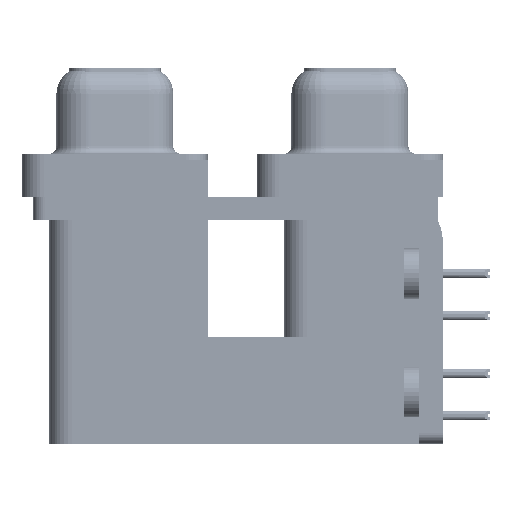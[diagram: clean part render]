
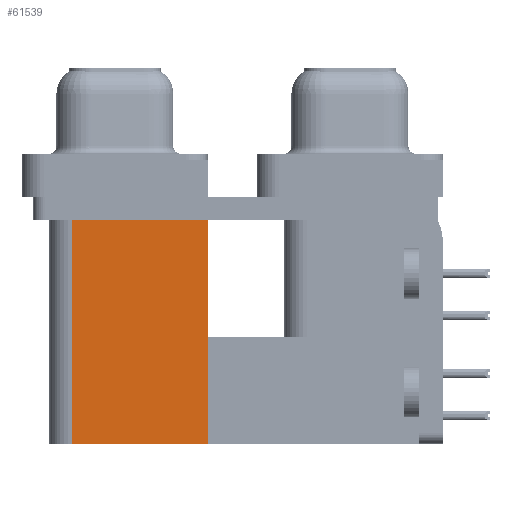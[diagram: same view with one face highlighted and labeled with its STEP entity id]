
A CAD part, left-side view. The second image highlights one B-rep face of the part: STEP entity #61539.
In plain terms, the highlighted planar face has unit normal (-1, 0, 0).
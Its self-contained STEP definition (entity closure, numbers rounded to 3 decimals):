
#267 = VECTOR ( 'NONE', #73419, 1000. ) ;
#1013 = CARTESIAN_POINT ( 'NONE',  ( 3.79, 18.8, -2.5 ) ) ;
#1048 = ORIENTED_EDGE ( 'NONE', *, *, #11530, .T. ) ;
#2386 = EDGE_CURVE ( 'NONE', #28716, #65193, #2513, .T. ) ;
#2513 = LINE ( 'NONE', #20990, #4728 ) ;
#4620 = VERTEX_POINT ( 'NONE', #12793 ) ;
#4728 = VECTOR ( 'NONE', #27381, 1000. ) ;
#11530 = EDGE_CURVE ( 'NONE', #44210, #65193, #68140, .T. ) ;
#12793 = CARTESIAN_POINT ( 'NONE',  ( 3.79, 9.6, -19.2 ) ) ;
#18564 = EDGE_CURVE ( 'NONE', #4620, #44210, #52692, .T. ) ;
#20990 = CARTESIAN_POINT ( 'NONE',  ( 3.79, 18.8, -19.2 ) ) ;
#21736 = DIRECTION ( 'NONE',  ( 1., 0., 0. ) ) ;
#27381 = DIRECTION ( 'NONE',  ( 0., 0., 1. ) ) ;
#28716 = VERTEX_POINT ( 'NONE', #68790 ) ;
#38647 = FACE_OUTER_BOUND ( 'NONE', #41746, .T. ) ;
#38941 = DIRECTION ( 'NONE',  ( 0., 1., 0. ) ) ;
#41746 = EDGE_LOOP ( 'NONE', ( #1048, #51373, #51739, #70966 ) ) ;
#44210 = VERTEX_POINT ( 'NONE', #59476 ) ;
#44662 = DIRECTION ( 'NONE',  ( 0., 0., -1. ) ) ;
#47395 = CARTESIAN_POINT ( 'NONE',  ( 3.79, 9.6, -19.2 ) ) ;
#49782 = VECTOR ( 'NONE', #38941, 1000. ) ;
#49881 = CARTESIAN_POINT ( 'NONE',  ( 3.79, 9.6, -19.2 ) ) ;
#50430 = CARTESIAN_POINT ( 'NONE',  ( 3.79, 9.6, -2.5 ) ) ;
#51373 = ORIENTED_EDGE ( 'NONE', *, *, #2386, .F. ) ;
#51739 = ORIENTED_EDGE ( 'NONE', *, *, #73454, .F. ) ;
#52692 = LINE ( 'NONE', #47395, #67981 ) ;
#55986 = CARTESIAN_POINT ( 'NONE',  ( 3.79, 9.6, -19.2 ) ) ;
#58094 = AXIS2_PLACEMENT_3D ( 'NONE', #55986, #21736, #44662 ) ;
#59476 = CARTESIAN_POINT ( 'NONE',  ( 3.79, 9.6, -2.5 ) ) ;
#61539 = ADVANCED_FACE ( 'NONE', ( #38647 ), #61624, .F. ) ;
#61624 = PLANE ( 'NONE',  #58094 ) ;
#65193 = VERTEX_POINT ( 'NONE', #1013 ) ;
#67981 = VECTOR ( 'NONE', #70377, 1000. ) ;
#68140 = LINE ( 'NONE', #50430, #267 ) ;
#68790 = CARTESIAN_POINT ( 'NONE',  ( 3.79, 18.8, -19.2 ) ) ;
#70377 = DIRECTION ( 'NONE',  ( 0., 0., 1. ) ) ;
#70966 = ORIENTED_EDGE ( 'NONE', *, *, #18564, .T. ) ;
#73419 = DIRECTION ( 'NONE',  ( 0., 1., 0. ) ) ;
#73454 = EDGE_CURVE ( 'NONE', #4620, #28716, #73602, .T. ) ;
#73602 = LINE ( 'NONE', #49881, #49782 ) ;
